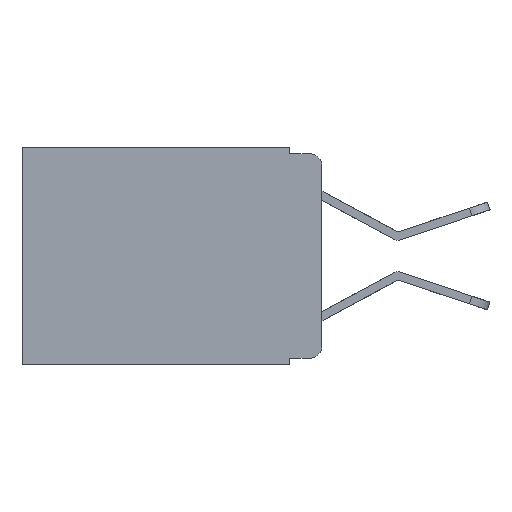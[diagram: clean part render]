
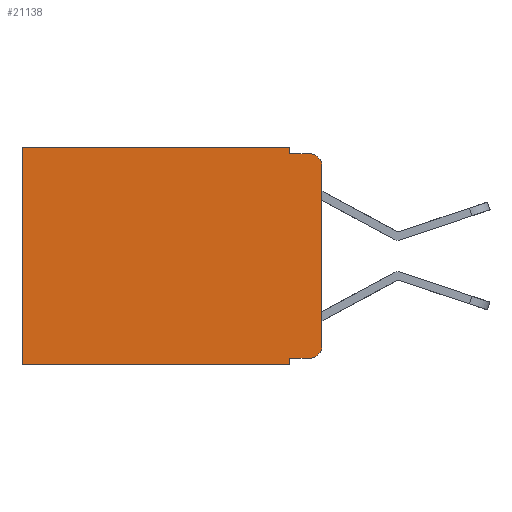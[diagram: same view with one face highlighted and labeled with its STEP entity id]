
A CAD part, left-side view. The second image highlights one B-rep face of the part: STEP entity #21138.
In plain terms, the highlighted planar face has unit normal (-1, 0, 0).
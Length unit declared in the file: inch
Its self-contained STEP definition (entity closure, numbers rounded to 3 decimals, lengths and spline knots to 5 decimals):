
#153 = VECTOR ( 'NONE', #23106, 39.37008 ) ;
#505 = CARTESIAN_POINT ( 'NONE',  ( 0.298, 0.051, 0. ) ) ;
#827 = CARTESIAN_POINT ( 'NONE',  ( 0.298, 0.02, -0.03 ) ) ;
#848 = EDGE_CURVE ( 'NONE', #11825, #20768, #5254, .T. ) ;
#1737 = LINE ( 'NONE', #17509, #16407 ) ;
#2260 = DIRECTION ( 'NONE',  ( 0., 0., -1. ) ) ;
#2422 = VERTEX_POINT ( 'NONE', #2454 ) ;
#2454 = CARTESIAN_POINT ( 'NONE',  ( 0.298, 0.051, 0. ) ) ;
#3042 = CARTESIAN_POINT ( 'NONE',  ( 0.298, 0.051, -0.333 ) ) ;
#3114 = VECTOR ( 'NONE', #23032, 39.37008 ) ;
#3133 = CARTESIAN_POINT ( 'NONE',  ( 0.298, 0.051, -0.01 ) ) ;
#4280 = VERTEX_POINT ( 'NONE', #24397 ) ;
#4369 = DIRECTION ( 'NONE',  ( 0., 0., -1. ) ) ;
#4596 = VECTOR ( 'NONE', #4369, 39.37008 ) ;
#4607 = EDGE_CURVE ( 'NONE', #14810, #6875, #16278, .T. ) ;
#5188 = LINE ( 'NONE', #11125, #3114 ) ;
#5254 = LINE ( 'NONE', #7739, #9954 ) ;
#5277 = CARTESIAN_POINT ( 'NONE',  ( 0.298, 0.02, -0.333 ) ) ;
#5387 = CARTESIAN_POINT ( 'NONE',  ( 0.298, 0.473, -0.343 ) ) ;
#5477 = CARTESIAN_POINT ( 'NONE',  ( 0.298, 0.051, -0.343 ) ) ;
#5955 = ORIENTED_EDGE ( 'NONE', *, *, #17031, .F. ) ;
#6120 = DIRECTION ( 'NONE',  ( 0., 0., -1. ) ) ;
#6466 = LINE ( 'NONE', #505, #4596 ) ;
#6875 = VERTEX_POINT ( 'NONE', #15857 ) ;
#7006 = EDGE_CURVE ( 'NONE', #2422, #4280, #7098, .T. ) ;
#7098 = LINE ( 'NONE', #19017, #17408 ) ;
#7534 = ORIENTED_EDGE ( 'NONE', *, *, #7006, .T. ) ;
#7720 = EDGE_CURVE ( 'NONE', #10795, #6875, #11016, .T. ) ;
#7739 = CARTESIAN_POINT ( 'NONE',  ( 0.298, 0., -0.343 ) ) ;
#8238 = DIRECTION ( 'NONE',  ( 0., -1., 0. ) ) ;
#8422 = CIRCLE ( 'NONE', #25327, 0.02 ) ;
#9691 = CARTESIAN_POINT ( 'NONE',  ( 0.298, 0., 0. ) ) ;
#9830 = ORIENTED_EDGE ( 'NONE', *, *, #24430, .T. ) ;
#9948 = CARTESIAN_POINT ( 'NONE',  ( 0.298, 0.02, -0.313 ) ) ;
#9954 = VECTOR ( 'NONE', #15818, 39.37008 ) ;
#10102 = LINE ( 'NONE', #18191, #19852 ) ;
#10325 = EDGE_CURVE ( 'NONE', #4280, #20768, #5188, .T. ) ;
#10795 = VERTEX_POINT ( 'NONE', #5277 ) ;
#11016 = CIRCLE ( 'NONE', #13135, 0.02 ) ;
#11125 = CARTESIAN_POINT ( 'NONE',  ( 0.298, 0.473, 0. ) ) ;
#11557 = DIRECTION ( 'NONE',  ( 1., 0., 0. ) ) ;
#11825 = VERTEX_POINT ( 'NONE', #5477 ) ;
#12443 = EDGE_CURVE ( 'NONE', #23970, #19722, #21250, .T. ) ;
#13115 = VECTOR ( 'NONE', #2260, 39.37008 ) ;
#13135 = AXIS2_PLACEMENT_3D ( 'NONE', #9948, #19894, #6120 ) ;
#14324 = EDGE_LOOP ( 'NONE', ( #25659, #9830, #21311, #5955, #7534, #24836, #25303, #15276, #18649, #21489 ) ) ;
#14810 = VERTEX_POINT ( 'NONE', #18434 ) ;
#15276 = ORIENTED_EDGE ( 'NONE', *, *, #22899, .F. ) ;
#15543 = AXIS2_PLACEMENT_3D ( 'NONE', #9691, #11557, #25446 ) ;
#15818 = DIRECTION ( 'NONE',  ( 0., 1., 0. ) ) ;
#15857 = CARTESIAN_POINT ( 'NONE',  ( 0.298, 0., -0.313 ) ) ;
#16278 = LINE ( 'NONE', #19997, #13115 ) ;
#16407 = VECTOR ( 'NONE', #25553, 39.37008 ) ;
#17031 = EDGE_CURVE ( 'NONE', #2422, #23970, #6466, .T. ) ;
#17177 = DIRECTION ( 'NONE',  ( 0., 1., 0. ) ) ;
#17408 = VECTOR ( 'NONE', #17177, 39.37008 ) ;
#17509 = CARTESIAN_POINT ( 'NONE',  ( 0.298, 0.051, 0. ) ) ;
#18191 = CARTESIAN_POINT ( 'NONE',  ( 0.298, 0.051, -0.333 ) ) ;
#18434 = CARTESIAN_POINT ( 'NONE',  ( 0.298, 0., -0.03 ) ) ;
#18649 = ORIENTED_EDGE ( 'NONE', *, *, #24338, .T. ) ;
#19017 = CARTESIAN_POINT ( 'NONE',  ( 0.298, 0., 0. ) ) ;
#19722 = VERTEX_POINT ( 'NONE', #25046 ) ;
#19852 = VECTOR ( 'NONE', #8238, 39.37008 ) ;
#19894 = DIRECTION ( 'NONE',  ( -1., 0., 0. ) ) ;
#19997 = CARTESIAN_POINT ( 'NONE',  ( 0.298, 0., 0. ) ) ;
#20211 = VERTEX_POINT ( 'NONE', #3042 ) ;
#20768 = VERTEX_POINT ( 'NONE', #5387 ) ;
#20821 = DIRECTION ( 'NONE',  ( 0., 0., -1. ) ) ;
#21138 = ADVANCED_FACE ( 'NONE', ( #24912 ), #23968, .F. ) ;
#21250 = LINE ( 'NONE', #3133, #153 ) ;
#21311 = ORIENTED_EDGE ( 'NONE', *, *, #12443, .F. ) ;
#21489 = ORIENTED_EDGE ( 'NONE', *, *, #7720, .T. ) ;
#22899 = EDGE_CURVE ( 'NONE', #20211, #11825, #1737, .T. ) ;
#23032 = DIRECTION ( 'NONE',  ( 0., 0., -1. ) ) ;
#23060 = DIRECTION ( 'NONE',  ( -1., 0., 0. ) ) ;
#23095 = CARTESIAN_POINT ( 'NONE',  ( 0.298, 0.051, -0.01 ) ) ;
#23106 = DIRECTION ( 'NONE',  ( 0., -1., 0. ) ) ;
#23968 = PLANE ( 'NONE',  #15543 ) ;
#23970 = VERTEX_POINT ( 'NONE', #23095 ) ;
#24338 = EDGE_CURVE ( 'NONE', #20211, #10795, #10102, .T. ) ;
#24397 = CARTESIAN_POINT ( 'NONE',  ( 0.298, 0.473, 0. ) ) ;
#24430 = EDGE_CURVE ( 'NONE', #14810, #19722, #8422, .T. ) ;
#24836 = ORIENTED_EDGE ( 'NONE', *, *, #10325, .T. ) ;
#24912 = FACE_OUTER_BOUND ( 'NONE', #14324, .T. ) ;
#25046 = CARTESIAN_POINT ( 'NONE',  ( 0.298, 0.02, -0.01 ) ) ;
#25303 = ORIENTED_EDGE ( 'NONE', *, *, #848, .F. ) ;
#25327 = AXIS2_PLACEMENT_3D ( 'NONE', #827, #23060, #20821 ) ;
#25446 = DIRECTION ( 'NONE',  ( 0., 0., -1. ) ) ;
#25553 = DIRECTION ( 'NONE',  ( 0., 0., -1. ) ) ;
#25659 = ORIENTED_EDGE ( 'NONE', *, *, #4607, .F. ) ;
